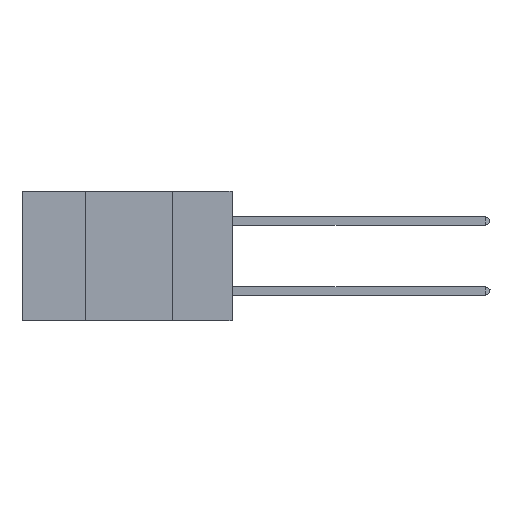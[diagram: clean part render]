
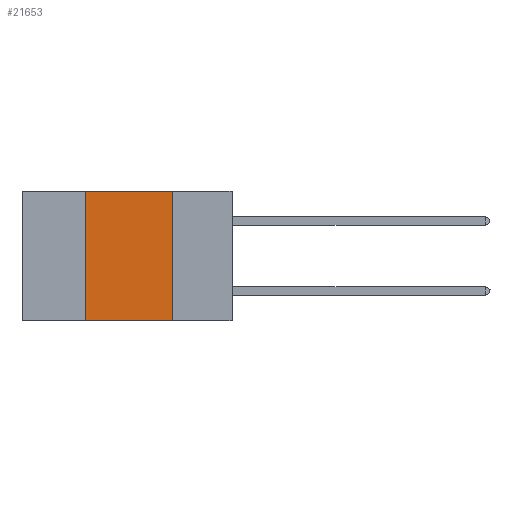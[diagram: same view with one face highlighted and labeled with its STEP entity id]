
A CAD part, left-side view. The second image highlights one B-rep face of the part: STEP entity #21653.
In plain terms, the highlighted planar face has unit normal (-1, 0, 0).
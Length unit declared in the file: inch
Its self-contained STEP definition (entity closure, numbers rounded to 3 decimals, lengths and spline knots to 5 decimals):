
#1588 = LINE ( 'NONE', #2686, #9037 ) ;
#2506 = ORIENTED_EDGE ( 'NONE', *, *, #21269, .F. ) ;
#2686 = CARTESIAN_POINT ( 'NONE',  ( 0., 0.6, -0.37 ) ) ;
#3096 = CARTESIAN_POINT ( 'NONE',  ( 0., 0.42, -0.37 ) ) ;
#3922 = VECTOR ( 'NONE', #14441, 39.37008 ) ;
#5356 = ORIENTED_EDGE ( 'NONE', *, *, #8157, .F. ) ;
#5576 = EDGE_CURVE ( 'NONE', #23246, #19820, #20047, .T. ) ;
#6021 = CARTESIAN_POINT ( 'NONE',  ( 0., 0.17, 0. ) ) ;
#6799 = DIRECTION ( 'NONE',  ( 0., 0., -1. ) ) ;
#7107 = AXIS2_PLACEMENT_3D ( 'NONE', #24422, #7286, #9837 ) ;
#7286 = DIRECTION ( 'NONE',  ( 1., 0., 0. ) ) ;
#7675 = EDGE_CURVE ( 'NONE', #20750, #21812, #1588, .T. ) ;
#8157 = EDGE_CURVE ( 'NONE', #20750, #23246, #20794, .T. ) ;
#8179 = CARTESIAN_POINT ( 'NONE',  ( 0., 0.17, -0.37 ) ) ;
#9037 = VECTOR ( 'NONE', #17833, 39.37008 ) ;
#9837 = DIRECTION ( 'NONE',  ( 0., 0., -1. ) ) ;
#10040 = ORIENTED_EDGE ( 'NONE', *, *, #7675, .T. ) ;
#11271 = PLANE ( 'NONE',  #7107 ) ;
#13826 = CARTESIAN_POINT ( 'NONE',  ( 0., 0.6, 0. ) ) ;
#14077 = DIRECTION ( 'NONE',  ( 0., -1., 0. ) ) ;
#14441 = DIRECTION ( 'NONE',  ( 0., 0., 1. ) ) ;
#16703 = VECTOR ( 'NONE', #6799, 39.37008 ) ;
#17459 = ORIENTED_EDGE ( 'NONE', *, *, #5576, .F. ) ;
#17833 = DIRECTION ( 'NONE',  ( 0., -1., 0. ) ) ;
#18199 = LINE ( 'NONE', #19822, #16703 ) ;
#18386 = CARTESIAN_POINT ( 'NONE',  ( 0., 0.42, 0. ) ) ;
#18448 = FACE_OUTER_BOUND ( 'NONE', #19927, .T. ) ;
#19820 = VERTEX_POINT ( 'NONE', #6021 ) ;
#19822 = CARTESIAN_POINT ( 'NONE',  ( 0., 0.17, 0. ) ) ;
#19927 = EDGE_LOOP ( 'NONE', ( #2506, #17459, #5356, #10040 ) ) ;
#20047 = LINE ( 'NONE', #13826, #24448 ) ;
#20750 = VERTEX_POINT ( 'NONE', #3096 ) ;
#20794 = LINE ( 'NONE', #18386, #3922 ) ;
#21269 = EDGE_CURVE ( 'NONE', #19820, #21812, #18199, .T. ) ;
#21653 = ADVANCED_FACE ( 'NONE', ( #18448 ), #11271, .F. ) ;
#21812 = VERTEX_POINT ( 'NONE', #8179 ) ;
#22745 = CARTESIAN_POINT ( 'NONE',  ( 0., 0.42, 0. ) ) ;
#23246 = VERTEX_POINT ( 'NONE', #22745 ) ;
#24422 = CARTESIAN_POINT ( 'NONE',  ( 0., 0.6, 0. ) ) ;
#24448 = VECTOR ( 'NONE', #14077, 39.37008 ) ;
